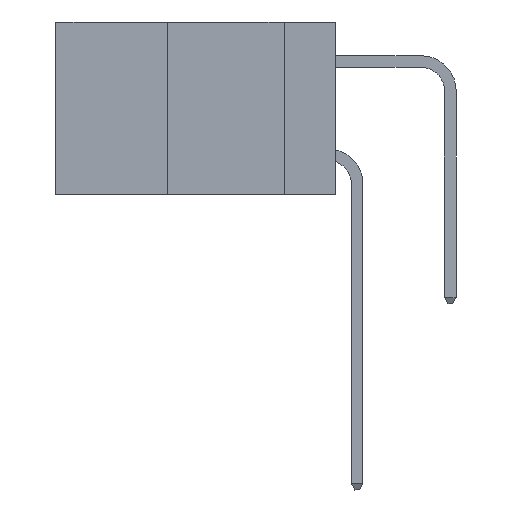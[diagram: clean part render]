
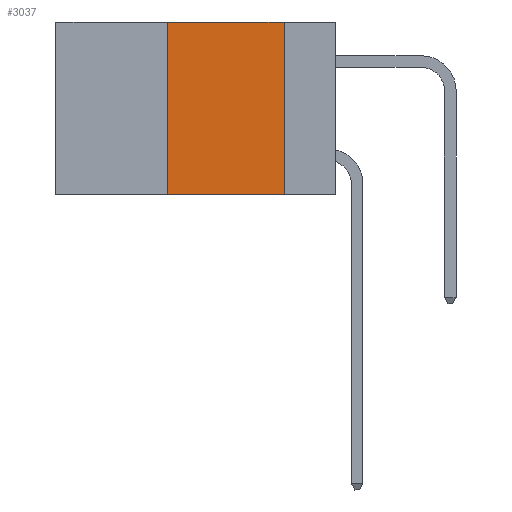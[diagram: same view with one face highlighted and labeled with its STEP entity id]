
A CAD part, left-side view. The second image highlights one B-rep face of the part: STEP entity #3037.
In plain terms, the highlighted planar face has unit normal (-1, 0, 0).
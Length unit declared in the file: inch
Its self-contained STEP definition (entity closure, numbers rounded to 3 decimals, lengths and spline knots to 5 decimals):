
#1379 = EDGE_CURVE ( 'NONE', #18256, #13596, #13347, .T. ) ;
#2417 = PLANE ( 'NONE',  #5485 ) ;
#2624 = VECTOR ( 'NONE', #9217, 39.37008 ) ;
#2810 = FACE_OUTER_BOUND ( 'NONE', #17634, .T. ) ;
#3037 = ADVANCED_FACE ( 'NONE', ( #2810 ), #2417, .F. ) ;
#3812 = DIRECTION ( 'NONE',  ( 1., 0., 0. ) ) ;
#4413 = DIRECTION ( 'NONE',  ( 0., 0., 1. ) ) ;
#5052 = ORIENTED_EDGE ( 'NONE', *, *, #15290, .T. ) ;
#5262 = VERTEX_POINT ( 'NONE', #9395 ) ;
#5485 = AXIS2_PLACEMENT_3D ( 'NONE', #19232, #3812, #10167 ) ;
#6201 = VECTOR ( 'NONE', #14166, 39.37008 ) ;
#8377 = EDGE_CURVE ( 'NONE', #16302, #18256, #15962, .T. ) ;
#9217 = DIRECTION ( 'NONE',  ( 0., -1., 0. ) ) ;
#9336 = LINE ( 'NONE', #15274, #2624 ) ;
#9395 = CARTESIAN_POINT ( 'NONE',  ( 0., 0.36, -0.37 ) ) ;
#9402 = CARTESIAN_POINT ( 'NONE',  ( 0., 0.11, 0. ) ) ;
#9497 = EDGE_CURVE ( 'NONE', #5262, #16302, #11141, .T. ) ;
#9542 = CARTESIAN_POINT ( 'NONE',  ( 0., 0.6, 0. ) ) ;
#10167 = DIRECTION ( 'NONE',  ( 0., 0., -1. ) ) ;
#10758 = VECTOR ( 'NONE', #15494, 39.37008 ) ;
#11141 = LINE ( 'NONE', #12796, #12087 ) ;
#11528 = ORIENTED_EDGE ( 'NONE', *, *, #9497, .F. ) ;
#12087 = VECTOR ( 'NONE', #4413, 39.37008 ) ;
#12796 = CARTESIAN_POINT ( 'NONE',  ( 0., 0.36, 0. ) ) ;
#13347 = LINE ( 'NONE', #18232, #10758 ) ;
#13596 = VERTEX_POINT ( 'NONE', #16371 ) ;
#14166 = DIRECTION ( 'NONE',  ( 0., -1., 0. ) ) ;
#15274 = CARTESIAN_POINT ( 'NONE',  ( 0., 0.6, -0.37 ) ) ;
#15290 = EDGE_CURVE ( 'NONE', #5262, #13596, #9336, .T. ) ;
#15494 = DIRECTION ( 'NONE',  ( 0., 0., -1. ) ) ;
#15962 = LINE ( 'NONE', #9542, #6201 ) ;
#16302 = VERTEX_POINT ( 'NONE', #17632 ) ;
#16371 = CARTESIAN_POINT ( 'NONE',  ( 0., 0.11, -0.37 ) ) ;
#17632 = CARTESIAN_POINT ( 'NONE',  ( 0., 0.36, 0. ) ) ;
#17634 = EDGE_LOOP ( 'NONE', ( #18064, #18257, #11528, #5052 ) ) ;
#18064 = ORIENTED_EDGE ( 'NONE', *, *, #1379, .F. ) ;
#18232 = CARTESIAN_POINT ( 'NONE',  ( 0., 0.11, 0. ) ) ;
#18256 = VERTEX_POINT ( 'NONE', #9402 ) ;
#18257 = ORIENTED_EDGE ( 'NONE', *, *, #8377, .F. ) ;
#19232 = CARTESIAN_POINT ( 'NONE',  ( 0., 0.6, 0. ) ) ;
